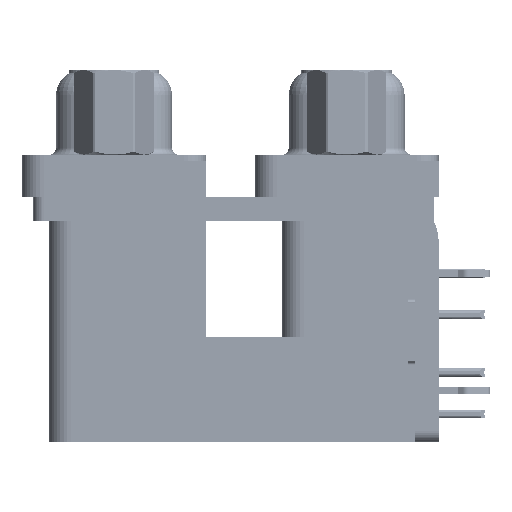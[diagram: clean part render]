
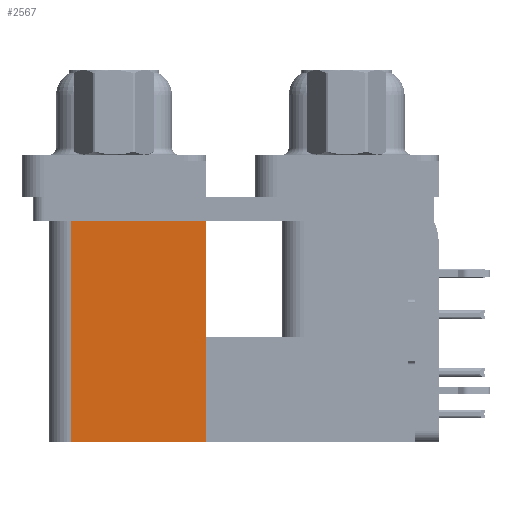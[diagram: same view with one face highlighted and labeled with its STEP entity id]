
A CAD part, left-side view. The second image highlights one B-rep face of the part: STEP entity #2567.
In plain terms, the highlighted planar face has unit normal (-1, 0, 0).
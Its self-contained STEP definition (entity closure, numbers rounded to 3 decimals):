
#599 = VECTOR ( 'NONE', #45415, 1000. ) ;
#1067 = CARTESIAN_POINT ( 'NONE',  ( 3.79, 18.8, -19.2 ) ) ;
#2567 = ADVANCED_FACE ( 'NONE', ( #7268 ), #32551, .F. ) ;
#3232 = EDGE_CURVE ( 'NONE', #18004, #52140, #38144, .T. ) ;
#4684 = ORIENTED_EDGE ( 'NONE', *, *, #80699, .T. ) ;
#7268 = FACE_OUTER_BOUND ( 'NONE', #71079, .T. ) ;
#8703 = AXIS2_PLACEMENT_3D ( 'NONE', #57822, #39580, #26342 ) ;
#14456 = LINE ( 'NONE', #19866, #46197 ) ;
#18004 = VERTEX_POINT ( 'NONE', #62187 ) ;
#18984 = VERTEX_POINT ( 'NONE', #77691 ) ;
#19866 = CARTESIAN_POINT ( 'NONE',  ( 3.79, 9.6, -19.2 ) ) ;
#20547 = VECTOR ( 'NONE', #77492, 1000. ) ;
#26342 = DIRECTION ( 'NONE',  ( 0., 0., -1. ) ) ;
#26754 = CARTESIAN_POINT ( 'NONE',  ( 3.79, 9.6, -19.2 ) ) ;
#32551 = PLANE ( 'NONE',  #8703 ) ;
#35182 = VERTEX_POINT ( 'NONE', #49439 ) ;
#38144 = LINE ( 'NONE', #63407, #20547 ) ;
#39580 = DIRECTION ( 'NONE',  ( 1., 0., 0. ) ) ;
#45415 = DIRECTION ( 'NONE',  ( 0., 0., 1. ) ) ;
#45559 = DIRECTION ( 'NONE',  ( 0., 1., 0. ) ) ;
#45820 = LINE ( 'NONE', #1067, #599 ) ;
#45982 = ORIENTED_EDGE ( 'NONE', *, *, #58681, .F. ) ;
#46197 = VECTOR ( 'NONE', #45559, 1000. ) ;
#49055 = VECTOR ( 'NONE', #52019, 1000. ) ;
#49439 = CARTESIAN_POINT ( 'NONE',  ( 3.79, 9.6, -19.2 ) ) ;
#52019 = DIRECTION ( 'NONE',  ( 0., 0., 1. ) ) ;
#52140 = VERTEX_POINT ( 'NONE', #66514 ) ;
#57822 = CARTESIAN_POINT ( 'NONE',  ( 3.79, 9.6, -19.2 ) ) ;
#58681 = EDGE_CURVE ( 'NONE', #18984, #52140, #45820, .T. ) ;
#62187 = CARTESIAN_POINT ( 'NONE',  ( 3.79, 9.6, -2.5 ) ) ;
#63407 = CARTESIAN_POINT ( 'NONE',  ( 3.79, 9.6, -2.5 ) ) ;
#63942 = ORIENTED_EDGE ( 'NONE', *, *, #76864, .F. ) ;
#64457 = LINE ( 'NONE', #26754, #49055 ) ;
#66514 = CARTESIAN_POINT ( 'NONE',  ( 3.79, 18.8, -2.5 ) ) ;
#71079 = EDGE_LOOP ( 'NONE', ( #78169, #45982, #63942, #4684 ) ) ;
#76864 = EDGE_CURVE ( 'NONE', #35182, #18984, #14456, .T. ) ;
#77492 = DIRECTION ( 'NONE',  ( 0., 1., 0. ) ) ;
#77691 = CARTESIAN_POINT ( 'NONE',  ( 3.79, 18.8, -19.2 ) ) ;
#78169 = ORIENTED_EDGE ( 'NONE', *, *, #3232, .T. ) ;
#80699 = EDGE_CURVE ( 'NONE', #35182, #18004, #64457, .T. ) ;
